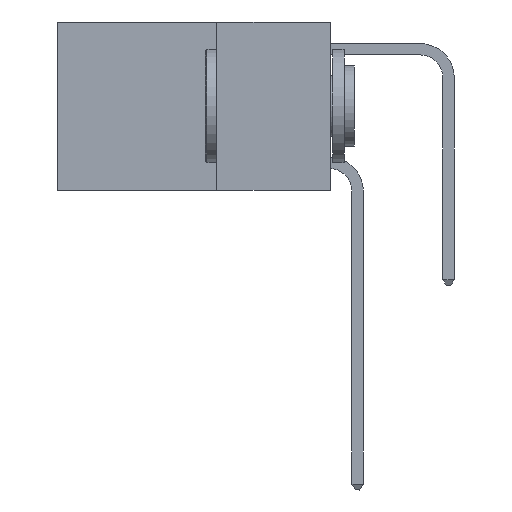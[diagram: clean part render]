
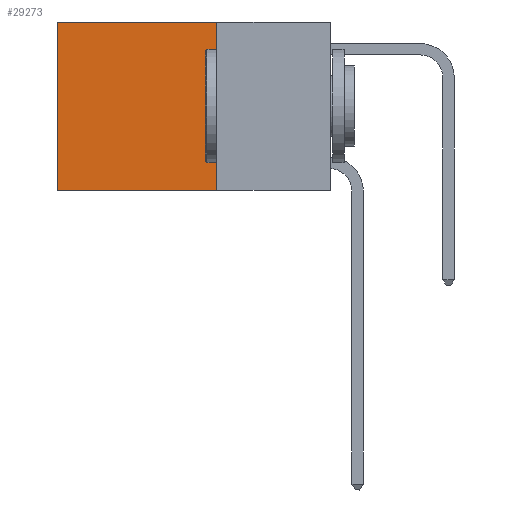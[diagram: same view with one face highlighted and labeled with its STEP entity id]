
A CAD part, left-side view. The second image highlights one B-rep face of the part: STEP entity #29273.
In plain terms, the highlighted planar face has unit normal (-1, 0, 0).
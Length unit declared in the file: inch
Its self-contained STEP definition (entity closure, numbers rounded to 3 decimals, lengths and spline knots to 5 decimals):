
#148 = DIRECTION ( 'NONE',  ( 0., 0., -1. ) ) ;
#529 = VECTOR ( 'NONE', #27970, 39.37008 ) ;
#1627 = CARTESIAN_POINT ( 'NONE',  ( 0.2625, 0.25, 0. ) ) ;
#1854 = ORIENTED_EDGE ( 'NONE', *, *, #25924, .T. ) ;
#2370 = DIRECTION ( 'NONE',  ( 1., 0., 0. ) ) ;
#2855 = LINE ( 'NONE', #7450, #13994 ) ;
#4418 = CARTESIAN_POINT ( 'NONE',  ( 0.2625, 0.25, 0. ) ) ;
#6491 = EDGE_CURVE ( 'NONE', #19336, #14447, #12030, .T. ) ;
#7096 = VECTOR ( 'NONE', #7222, 39.37008 ) ;
#7222 = DIRECTION ( 'NONE',  ( 0., 0., -1. ) ) ;
#7450 = CARTESIAN_POINT ( 'NONE',  ( 0.2625, 0.25, -0.37 ) ) ;
#7680 = AXIS2_PLACEMENT_3D ( 'NONE', #4418, #2370, #148 ) ;
#7980 = EDGE_LOOP ( 'NONE', ( #28233, #12931, #10830, #1854 ) ) ;
#10830 = ORIENTED_EDGE ( 'NONE', *, *, #21069, .F. ) ;
#12030 = LINE ( 'NONE', #31078, #15174 ) ;
#12931 = ORIENTED_EDGE ( 'NONE', *, *, #17524, .F. ) ;
#13994 = VECTOR ( 'NONE', #15203, 39.37008 ) ;
#14447 = VERTEX_POINT ( 'NONE', #17402 ) ;
#15174 = VECTOR ( 'NONE', #23937, 39.37008 ) ;
#15203 = DIRECTION ( 'NONE',  ( 0., 1., 0. ) ) ;
#16396 = CARTESIAN_POINT ( 'NONE',  ( 0.2625, 0.25, -0.37 ) ) ;
#16411 = VERTEX_POINT ( 'NONE', #20051 ) ;
#16757 = LINE ( 'NONE', #21353, #7096 ) ;
#17402 = CARTESIAN_POINT ( 'NONE',  ( 0.2625, 0.6, -0.37 ) ) ;
#17524 = EDGE_CURVE ( 'NONE', #26993, #14447, #2855, .T. ) ;
#19178 = CARTESIAN_POINT ( 'NONE',  ( 0.2625, 0.6, 0. ) ) ;
#19336 = VERTEX_POINT ( 'NONE', #19178 ) ;
#20051 = CARTESIAN_POINT ( 'NONE',  ( 0.2625, 0.25, 0. ) ) ;
#21069 = EDGE_CURVE ( 'NONE', #16411, #26993, #16757, .T. ) ;
#21353 = CARTESIAN_POINT ( 'NONE',  ( 0.2625, 0.25, 0. ) ) ;
#23937 = DIRECTION ( 'NONE',  ( 0., 0., -1. ) ) ;
#25924 = EDGE_CURVE ( 'NONE', #16411, #19336, #30195, .T. ) ;
#26180 = PLANE ( 'NONE',  #7680 ) ;
#26993 = VERTEX_POINT ( 'NONE', #16396 ) ;
#27970 = DIRECTION ( 'NONE',  ( 0., 1., 0. ) ) ;
#28233 = ORIENTED_EDGE ( 'NONE', *, *, #6491, .T. ) ;
#28881 = FACE_OUTER_BOUND ( 'NONE', #7980, .T. ) ;
#29273 = ADVANCED_FACE ( 'NONE', ( #28881 ), #26180, .F. ) ;
#30195 = LINE ( 'NONE', #1627, #529 ) ;
#31078 = CARTESIAN_POINT ( 'NONE',  ( 0.2625, 0.6, 0. ) ) ;
